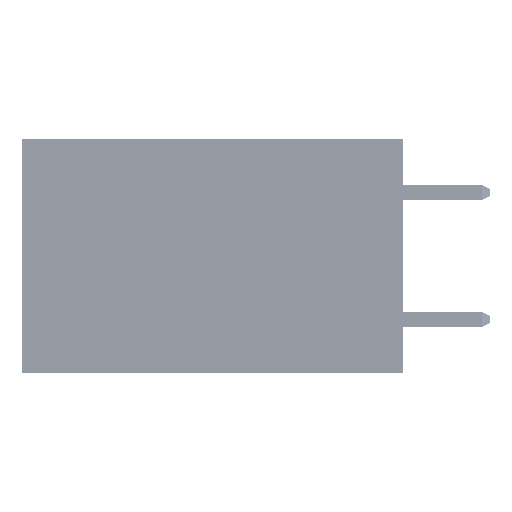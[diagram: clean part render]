
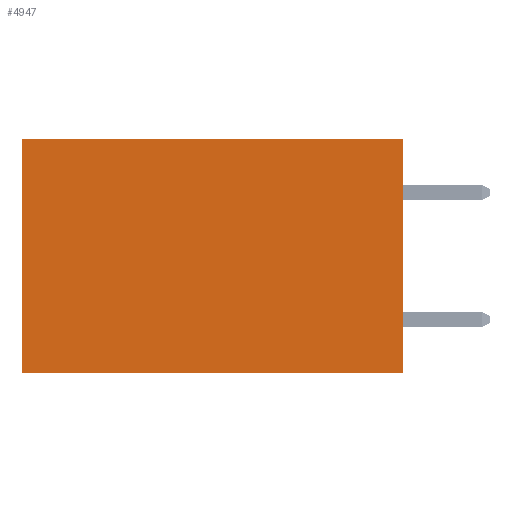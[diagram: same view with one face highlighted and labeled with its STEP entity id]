
A CAD part, left-side view. The second image highlights one B-rep face of the part: STEP entity #4947.
In plain terms, the highlighted planar face has unit normal (-1, 0, 0).
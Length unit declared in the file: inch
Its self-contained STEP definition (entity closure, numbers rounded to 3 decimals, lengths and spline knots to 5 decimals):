
#474 = VECTOR ( 'NONE', #17934, 39.37008 ) ;
#3666 = CARTESIAN_POINT ( 'NONE',  ( 0.2875, 0., 0. ) ) ;
#3830 = DIRECTION ( 'NONE',  ( 1., 0., 0. ) ) ;
#4701 = ORIENTED_EDGE ( 'NONE', *, *, #25494, .T. ) ;
#4947 = ADVANCED_FACE ( 'NONE', ( #24939 ), #22474, .F. ) ;
#5881 = CARTESIAN_POINT ( 'NONE',  ( 0.2875, 0.6, -0.37 ) ) ;
#5999 = ORIENTED_EDGE ( 'NONE', *, *, #21573, .T. ) ;
#7109 = VECTOR ( 'NONE', #40388, 39.37008 ) ;
#7543 = DIRECTION ( 'NONE',  ( 0., 0., -1. ) ) ;
#7555 = CARTESIAN_POINT ( 'NONE',  ( 0.2875, 0., 0. ) ) ;
#8283 = VERTEX_POINT ( 'NONE', #9069 ) ;
#9069 = CARTESIAN_POINT ( 'NONE',  ( 0.2875, 0.6, 0. ) ) ;
#14596 = LINE ( 'NONE', #47295, #22648 ) ;
#17934 = DIRECTION ( 'NONE',  ( 0., 0., -1. ) ) ;
#18039 = CARTESIAN_POINT ( 'NONE',  ( 0.2875, 0., -0.37 ) ) ;
#18246 = CARTESIAN_POINT ( 'NONE',  ( 0.2875, 0., -0.37 ) ) ;
#19904 = VERTEX_POINT ( 'NONE', #18246 ) ;
#19991 = ORIENTED_EDGE ( 'NONE', *, *, #30335, .F. ) ;
#20050 = LINE ( 'NONE', #28833, #474 ) ;
#20323 = CARTESIAN_POINT ( 'NONE',  ( 0.2875, 0., 0. ) ) ;
#21257 = DIRECTION ( 'NONE',  ( 0., 0., -1. ) ) ;
#21573 = EDGE_CURVE ( 'NONE', #38229, #8283, #43131, .T. ) ;
#22054 = LINE ( 'NONE', #18039, #7109 ) ;
#22474 = PLANE ( 'NONE',  #32019 ) ;
#22648 = VECTOR ( 'NONE', #21257, 39.37008 ) ;
#24105 = VERTEX_POINT ( 'NONE', #5881 ) ;
#24939 = FACE_OUTER_BOUND ( 'NONE', #45427, .T. ) ;
#25494 = EDGE_CURVE ( 'NONE', #8283, #24105, #20050, .T. ) ;
#28833 = CARTESIAN_POINT ( 'NONE',  ( 0.2875, 0.6, 0. ) ) ;
#29615 = ORIENTED_EDGE ( 'NONE', *, *, #30466, .F. ) ;
#30335 = EDGE_CURVE ( 'NONE', #38229, #19904, #14596, .T. ) ;
#30466 = EDGE_CURVE ( 'NONE', #19904, #24105, #22054, .T. ) ;
#32019 = AXIS2_PLACEMENT_3D ( 'NONE', #3666, #3830, #7543 ) ;
#37768 = DIRECTION ( 'NONE',  ( 0., 1., 0. ) ) ;
#38229 = VERTEX_POINT ( 'NONE', #20323 ) ;
#40388 = DIRECTION ( 'NONE',  ( 0., 1., 0. ) ) ;
#43131 = LINE ( 'NONE', #7555, #46523 ) ;
#45427 = EDGE_LOOP ( 'NONE', ( #4701, #29615, #19991, #5999 ) ) ;
#46523 = VECTOR ( 'NONE', #37768, 39.37008 ) ;
#47295 = CARTESIAN_POINT ( 'NONE',  ( 0.2875, 0., 0. ) ) ;
